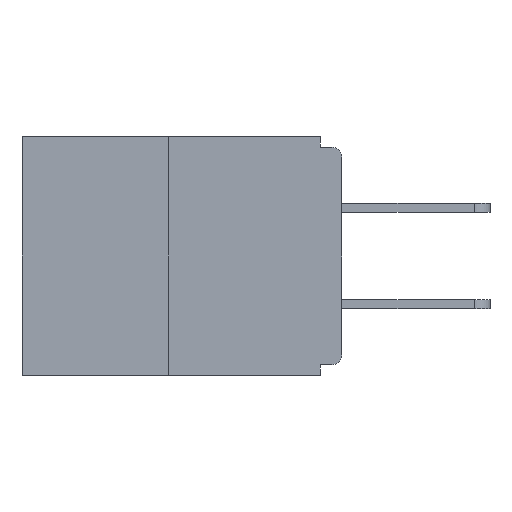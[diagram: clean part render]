
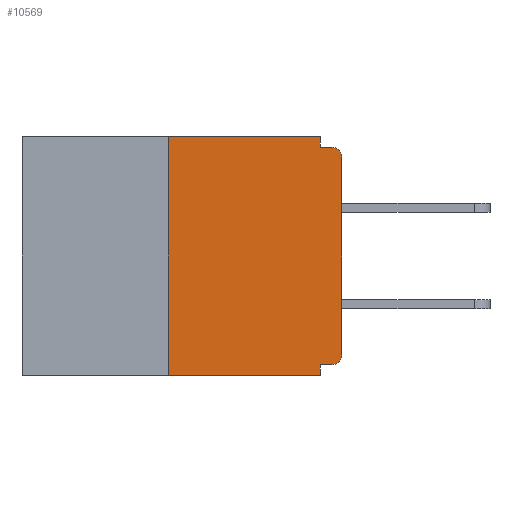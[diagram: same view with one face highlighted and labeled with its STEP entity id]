
A CAD part, left-side view. The second image highlights one B-rep face of the part: STEP entity #10569.
In plain terms, the highlighted planar face has unit normal (-1, 0, 0).
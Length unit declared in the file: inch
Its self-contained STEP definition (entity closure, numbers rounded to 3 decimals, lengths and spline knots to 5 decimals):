
#38 = ORIENTED_EDGE ( 'NONE', *, *, #6070, .T. ) ;
#615 = EDGE_CURVE ( 'NONE', #7480, #11507, #5661, .T. ) ;
#890 = EDGE_CURVE ( 'NONE', #9545, #17330, #10823, .T. ) ;
#917 = CARTESIAN_POINT ( 'NONE',  ( 0., 0.015, -0.03 ) ) ;
#919 = ORIENTED_EDGE ( 'NONE', *, *, #2862, .T. ) ;
#1250 = DIRECTION ( 'NONE',  ( 0., 0., -1. ) ) ;
#2083 = ORIENTED_EDGE ( 'NONE', *, *, #615, .F. ) ;
#2160 = VECTOR ( 'NONE', #9314, 39.37008 ) ;
#2420 = VERTEX_POINT ( 'NONE', #12390 ) ;
#2480 = CIRCLE ( 'NONE', #16948, 0.015 ) ;
#2862 = EDGE_CURVE ( 'NONE', #11780, #7326, #17047, .T. ) ;
#2921 = CARTESIAN_POINT ( 'NONE',  ( 0., 0.031, -0.328 ) ) ;
#2951 = ORIENTED_EDGE ( 'NONE', *, *, #20837, .T. ) ;
#3122 = LINE ( 'NONE', #12594, #19189 ) ;
#3250 = EDGE_LOOP ( 'NONE', ( #2083, #13430, #919, #19632, #12050, #2951, #14568, #38, #19454, #15542 ) ) ;
#3474 = DIRECTION ( 'NONE',  ( 0., -1., 0. ) ) ;
#3712 = CARTESIAN_POINT ( 'NONE',  ( 0., 0.015, -0.015 ) ) ;
#3949 = EDGE_CURVE ( 'NONE', #11507, #2420, #13815, .T. ) ;
#4074 = CARTESIAN_POINT ( 'NONE',  ( 0., 0., -0.313 ) ) ;
#4269 = AXIS2_PLACEMENT_3D ( 'NONE', #19511, #9079, #10840 ) ;
#5420 = VERTEX_POINT ( 'NONE', #3712 ) ;
#5585 = PLANE ( 'NONE',  #4269 ) ;
#5625 = CARTESIAN_POINT ( 'NONE',  ( 0., 0.25, 0. ) ) ;
#5661 = LINE ( 'NONE', #8022, #13246 ) ;
#5921 = CARTESIAN_POINT ( 'NONE',  ( 0., 0., -0.328 ) ) ;
#6047 = LINE ( 'NONE', #17769, #6870 ) ;
#6070 = EDGE_CURVE ( 'NONE', #8721, #5420, #11334, .T. ) ;
#6089 = EDGE_CURVE ( 'NONE', #8525, #8721, #20039, .T. ) ;
#6214 = AXIS2_PLACEMENT_3D ( 'NONE', #917, #13046, #14820 ) ;
#6627 = EDGE_CURVE ( 'NONE', #2420, #5420, #3122, .T. ) ;
#6870 = VECTOR ( 'NONE', #19507, 39.37008 ) ;
#7017 = CARTESIAN_POINT ( 'NONE',  ( 0., 0., -0.03 ) ) ;
#7326 = VERTEX_POINT ( 'NONE', #16343 ) ;
#7480 = VERTEX_POINT ( 'NONE', #12111 ) ;
#8022 = CARTESIAN_POINT ( 'NONE',  ( 0., 0.46, 0. ) ) ;
#8525 = VERTEX_POINT ( 'NONE', #4074 ) ;
#8607 = VECTOR ( 'NONE', #3474, 39.37008 ) ;
#8721 = VERTEX_POINT ( 'NONE', #7017 ) ;
#9040 = DIRECTION ( 'NONE',  ( 0., 0., 1. ) ) ;
#9079 = DIRECTION ( 'NONE',  ( 1., 0., 0. ) ) ;
#9314 = DIRECTION ( 'NONE',  ( 0., 0., -1. ) ) ;
#9545 = VERTEX_POINT ( 'NONE', #18131 ) ;
#9630 = DIRECTION ( 'NONE',  ( 0., 0., 1. ) ) ;
#9742 = DIRECTION ( 'NONE',  ( 0., -1., 0. ) ) ;
#9971 = DIRECTION ( 'NONE',  ( -1., 0., 0. ) ) ;
#10569 = ADVANCED_FACE ( 'NONE', ( #19829 ), #5585, .F. ) ;
#10823 = LINE ( 'NONE', #5921, #15698 ) ;
#10840 = DIRECTION ( 'NONE',  ( 0., 0., -1. ) ) ;
#11334 = CIRCLE ( 'NONE', #6214, 0.015 ) ;
#11507 = VERTEX_POINT ( 'NONE', #16324 ) ;
#11633 = CARTESIAN_POINT ( 'NONE',  ( 0., 0.015, -0.313 ) ) ;
#11780 = VERTEX_POINT ( 'NONE', #19564 ) ;
#12050 = ORIENTED_EDGE ( 'NONE', *, *, #890, .F. ) ;
#12111 = CARTESIAN_POINT ( 'NONE',  ( 0., 0.25, 0. ) ) ;
#12390 = CARTESIAN_POINT ( 'NONE',  ( 0., 0.031, -0.015 ) ) ;
#12594 = CARTESIAN_POINT ( 'NONE',  ( 0., 0., -0.015 ) ) ;
#12969 = CARTESIAN_POINT ( 'NONE',  ( 0., 0., 0. ) ) ;
#13046 = DIRECTION ( 'NONE',  ( -1., 0., 0. ) ) ;
#13246 = VECTOR ( 'NONE', #9742, 39.37008 ) ;
#13430 = ORIENTED_EDGE ( 'NONE', *, *, #21364, .F. ) ;
#13815 = LINE ( 'NONE', #16231, #2160 ) ;
#13859 = CARTESIAN_POINT ( 'NONE',  ( 0., 0.46, -0.343 ) ) ;
#14568 = ORIENTED_EDGE ( 'NONE', *, *, #6089, .T. ) ;
#14820 = DIRECTION ( 'NONE',  ( 0., 0., -1. ) ) ;
#14922 = EDGE_CURVE ( 'NONE', #17330, #7326, #6047, .T. ) ;
#15542 = ORIENTED_EDGE ( 'NONE', *, *, #3949, .F. ) ;
#15674 = VECTOR ( 'NONE', #9630, 39.37008 ) ;
#15698 = VECTOR ( 'NONE', #16484, 39.37008 ) ;
#16231 = CARTESIAN_POINT ( 'NONE',  ( 0., 0.031, 0. ) ) ;
#16324 = CARTESIAN_POINT ( 'NONE',  ( 0., 0.031, 0. ) ) ;
#16343 = CARTESIAN_POINT ( 'NONE',  ( 0., 0.031, -0.343 ) ) ;
#16484 = DIRECTION ( 'NONE',  ( 0., 1., 0. ) ) ;
#16948 = AXIS2_PLACEMENT_3D ( 'NONE', #11633, #9971, #1250 ) ;
#17047 = LINE ( 'NONE', #13859, #8607 ) ;
#17330 = VERTEX_POINT ( 'NONE', #2921 ) ;
#17673 = VECTOR ( 'NONE', #9040, 39.37008 ) ;
#17769 = CARTESIAN_POINT ( 'NONE',  ( 0., 0.031, -0.343 ) ) ;
#18131 = CARTESIAN_POINT ( 'NONE',  ( 0., 0.015, -0.328 ) ) ;
#18494 = LINE ( 'NONE', #5625, #17673 ) ;
#19189 = VECTOR ( 'NONE', #21119, 39.37008 ) ;
#19454 = ORIENTED_EDGE ( 'NONE', *, *, #6627, .F. ) ;
#19507 = DIRECTION ( 'NONE',  ( 0., 0., -1. ) ) ;
#19511 = CARTESIAN_POINT ( 'NONE',  ( 0., 0.46, 0. ) ) ;
#19564 = CARTESIAN_POINT ( 'NONE',  ( 0., 0.25, -0.343 ) ) ;
#19632 = ORIENTED_EDGE ( 'NONE', *, *, #14922, .F. ) ;
#19829 = FACE_OUTER_BOUND ( 'NONE', #3250, .T. ) ;
#20039 = LINE ( 'NONE', #12969, #15674 ) ;
#20837 = EDGE_CURVE ( 'NONE', #9545, #8525, #2480, .T. ) ;
#21119 = DIRECTION ( 'NONE',  ( 0., -1., 0. ) ) ;
#21364 = EDGE_CURVE ( 'NONE', #11780, #7480, #18494, .T. ) ;
